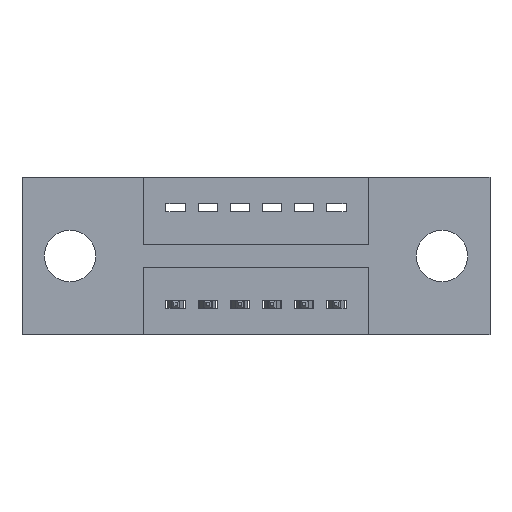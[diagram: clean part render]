
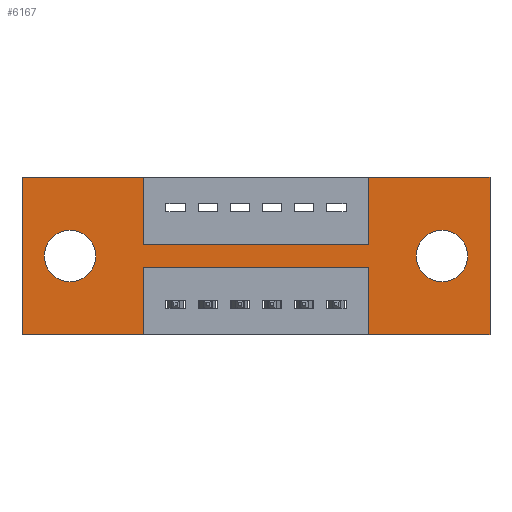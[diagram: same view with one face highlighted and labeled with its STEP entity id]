
A CAD part, front view. The second image highlights one B-rep face of the part: STEP entity #6167.
In plain terms, the highlighted planar face has unit normal (0, -1, 0).
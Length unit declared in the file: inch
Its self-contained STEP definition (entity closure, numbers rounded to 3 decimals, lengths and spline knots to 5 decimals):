
#45 = AXIS2_PLACEMENT_3D ( 'NONE', #7279, #2734, #5345 ) ;
#83 = CARTESIAN_POINT ( 'NONE',  ( 1.455, 0., 0. ) ) ;
#121 = ORIENTED_EDGE ( 'NONE', *, *, #7552, .F. ) ;
#159 = VECTOR ( 'NONE', #7605, 39.37008 ) ;
#226 = CARTESIAN_POINT ( 'NONE',  ( 1.0775, 0., -0.28 ) ) ;
#265 = FACE_BOUND ( 'NONE', #7285, .T. ) ;
#382 = CIRCLE ( 'NONE', #4432, 0.08 ) ;
#390 = ORIENTED_EDGE ( 'NONE', *, *, #767, .F. ) ;
#437 = ORIENTED_EDGE ( 'NONE', *, *, #5934, .F. ) ;
#606 = DIRECTION ( 'NONE',  ( 0., 0., 1. ) ) ;
#667 = DIRECTION ( 'NONE',  ( 0., 1., 0. ) ) ;
#767 = EDGE_CURVE ( 'NONE', #7581, #5680, #3666, .T. ) ;
#814 = ORIENTED_EDGE ( 'NONE', *, *, #2601, .F. ) ;
#1034 = CARTESIAN_POINT ( 'NONE',  ( 0.3775, 0., -0.21 ) ) ;
#1051 = PLANE ( 'NONE',  #6440 ) ;
#1087 = VERTEX_POINT ( 'NONE', #6138 ) ;
#1097 = DIRECTION ( 'NONE',  ( 0., 0., -1. ) ) ;
#1158 = DIRECTION ( 'NONE',  ( -1., 0., 0. ) ) ;
#1218 = ORIENTED_EDGE ( 'NONE', *, *, #6823, .F. ) ;
#1229 = VECTOR ( 'NONE', #1097, 39.37008 ) ;
#1241 = VECTOR ( 'NONE', #2586, 39.37008 ) ;
#1243 = VECTOR ( 'NONE', #2256, 39.37008 ) ;
#1257 = VECTOR ( 'NONE', #1158, 39.37008 ) ;
#1341 = EDGE_CURVE ( 'NONE', #1511, #5667, #7652, .T. ) ;
#1365 = CARTESIAN_POINT ( 'NONE',  ( 0.3775, 0., -0.49 ) ) ;
#1400 = DIRECTION ( 'NONE',  ( 0., 0., -1. ) ) ;
#1401 = VERTEX_POINT ( 'NONE', #8086 ) ;
#1511 = VERTEX_POINT ( 'NONE', #7092 ) ;
#1522 = DIRECTION ( 'NONE',  ( 0., 0., 1. ) ) ;
#1617 = VERTEX_POINT ( 'NONE', #7292 ) ;
#1715 = ORIENTED_EDGE ( 'NONE', *, *, #3439, .F. ) ;
#1744 = CARTESIAN_POINT ( 'NONE',  ( 0.1495, 0., -0.325 ) ) ;
#1856 = LINE ( 'NONE', #2813, #1243 ) ;
#1900 = LINE ( 'NONE', #2518, #1241 ) ;
#1903 = DIRECTION ( 'NONE',  ( 0., 0., -1. ) ) ;
#2095 = ORIENTED_EDGE ( 'NONE', *, *, #2577, .F. ) ;
#2156 = ORIENTED_EDGE ( 'NONE', *, *, #5410, .T. ) ;
#2192 = CIRCLE ( 'NONE', #5036, 0.08 ) ;
#2193 = CARTESIAN_POINT ( 'NONE',  ( 0.3775, 0., -0.21 ) ) ;
#2198 = CARTESIAN_POINT ( 'NONE',  ( 0., 0., 0. ) ) ;
#2256 = DIRECTION ( 'NONE',  ( -1., 0., 0. ) ) ;
#2380 = ORIENTED_EDGE ( 'NONE', *, *, #4853, .T. ) ;
#2443 = CARTESIAN_POINT ( 'NONE',  ( 1.0775, 0., -0.21 ) ) ;
#2518 = CARTESIAN_POINT ( 'NONE',  ( 0.3775, 0., -0.28 ) ) ;
#2527 = CARTESIAN_POINT ( 'NONE',  ( 0., 0., -0.49 ) ) ;
#2567 = LINE ( 'NONE', #2527, #6413 ) ;
#2577 = EDGE_CURVE ( 'NONE', #7084, #5293, #3788, .T. ) ;
#2586 = DIRECTION ( 'NONE',  ( 0., 0., -1. ) ) ;
#2598 = ORIENTED_EDGE ( 'NONE', *, *, #1341, .F. ) ;
#2601 = EDGE_CURVE ( 'NONE', #2740, #7581, #5428, .T. ) ;
#2621 = EDGE_LOOP ( 'NONE', ( #390, #814, #7301, #2862, #2598, #437, #121, #5266, #2095, #1715, #1218, #3570 ) ) ;
#2734 = DIRECTION ( 'NONE',  ( 0., 1., 0. ) ) ;
#2740 = VERTEX_POINT ( 'NONE', #1034 ) ;
#2776 = FACE_BOUND ( 'NONE', #6058, .T. ) ;
#2813 = CARTESIAN_POINT ( 'NONE',  ( 0.3775, 0., -0.28 ) ) ;
#2862 = ORIENTED_EDGE ( 'NONE', *, *, #6723, .F. ) ;
#2925 = ORIENTED_EDGE ( 'NONE', *, *, #5354, .T. ) ;
#3052 = VERTEX_POINT ( 'NONE', #1365 ) ;
#3074 = DIRECTION ( 'NONE',  ( 1., 0., 0. ) ) ;
#3151 = CARTESIAN_POINT ( 'NONE',  ( 0.1495, 0., -0.245 ) ) ;
#3234 = VERTEX_POINT ( 'NONE', #4937 ) ;
#3439 = EDGE_CURVE ( 'NONE', #6186, #7084, #2567, .T. ) ;
#3562 = VERTEX_POINT ( 'NONE', #4065 ) ;
#3570 = ORIENTED_EDGE ( 'NONE', *, *, #5876, .F. ) ;
#3621 = CIRCLE ( 'NONE', #45, 0.08 ) ;
#3666 = LINE ( 'NONE', #2443, #6799 ) ;
#3691 = VECTOR ( 'NONE', #3074, 39.37008 ) ;
#3788 = LINE ( 'NONE', #226, #7334 ) ;
#3817 = CARTESIAN_POINT ( 'NONE',  ( 0.1495, 0., -0.245 ) ) ;
#4065 = CARTESIAN_POINT ( 'NONE',  ( 1.3055, 0., -0.165 ) ) ;
#4267 = CARTESIAN_POINT ( 'NONE',  ( 0., 0., -0.49 ) ) ;
#4326 = AXIS2_PLACEMENT_3D ( 'NONE', #3817, #667, #5806 ) ;
#4333 = EDGE_CURVE ( 'NONE', #3562, #5982, #3621, .T. ) ;
#4432 = AXIS2_PLACEMENT_3D ( 'NONE', #3151, #7658, #606 ) ;
#4745 = CARTESIAN_POINT ( 'NONE',  ( 0., 0., 0. ) ) ;
#4789 = VERTEX_POINT ( 'NONE', #1744 ) ;
#4853 = EDGE_CURVE ( 'NONE', #5982, #3562, #2192, .T. ) ;
#4937 = CARTESIAN_POINT ( 'NONE',  ( 0.3775, 0., -0.28 ) ) ;
#5036 = AXIS2_PLACEMENT_3D ( 'NONE', #7853, #5084, #1400 ) ;
#5084 = DIRECTION ( 'NONE',  ( 0., 1., 0. ) ) ;
#5088 = VECTOR ( 'NONE', #1903, 39.37008 ) ;
#5141 = CARTESIAN_POINT ( 'NONE',  ( 1.3055, 0., -0.325 ) ) ;
#5266 = ORIENTED_EDGE ( 'NONE', *, *, #6476, .F. ) ;
#5293 = VERTEX_POINT ( 'NONE', #5736 ) ;
#5296 = LINE ( 'NONE', #83, #5088 ) ;
#5310 = LINE ( 'NONE', #6960, #159 ) ;
#5345 = DIRECTION ( 'NONE',  ( 0., 0., -1. ) ) ;
#5354 = EDGE_CURVE ( 'NONE', #1401, #4789, #8151, .T. ) ;
#5410 = EDGE_CURVE ( 'NONE', #4789, #1401, #382, .T. ) ;
#5428 = LINE ( 'NONE', #2193, #6622 ) ;
#5644 = CARTESIAN_POINT ( 'NONE',  ( 0., 0., 0. ) ) ;
#5667 = VERTEX_POINT ( 'NONE', #2198 ) ;
#5680 = VERTEX_POINT ( 'NONE', #6721 ) ;
#5736 = CARTESIAN_POINT ( 'NONE',  ( 1.0775, 0., -0.28 ) ) ;
#5806 = DIRECTION ( 'NONE',  ( 0., 0., 1. ) ) ;
#5814 = LINE ( 'NONE', #5644, #3691 ) ;
#5876 = EDGE_CURVE ( 'NONE', #5680, #1617, #5814, .T. ) ;
#5878 = DIRECTION ( 'NONE',  ( -1., 0., 0. ) ) ;
#5902 = DIRECTION ( 'NONE',  ( 0., 0., 1. ) ) ;
#5934 = EDGE_CURVE ( 'NONE', #3052, #1511, #7730, .T. ) ;
#5982 = VERTEX_POINT ( 'NONE', #5141 ) ;
#6058 = EDGE_LOOP ( 'NONE', ( #2925, #2156 ) ) ;
#6138 = CARTESIAN_POINT ( 'NONE',  ( 0.3775, 0., 0. ) ) ;
#6167 = ADVANCED_FACE ( 'NONE', ( #265, #2776, #6720 ), #1051, .T. ) ;
#6186 = VERTEX_POINT ( 'NONE', #7437 ) ;
#6191 = DIRECTION ( 'NONE',  ( 0., 0., -1. ) ) ;
#6313 = ORIENTED_EDGE ( 'NONE', *, *, #4333, .T. ) ;
#6413 = VECTOR ( 'NONE', #5878, 39.37008 ) ;
#6440 = AXIS2_PLACEMENT_3D ( 'NONE', #4267, #6864, #6191 ) ;
#6476 = EDGE_CURVE ( 'NONE', #5293, #3234, #1856, .T. ) ;
#6622 = VECTOR ( 'NONE', #7419, 39.37008 ) ;
#6657 = DIRECTION ( 'NONE',  ( 0., 0., 1. ) ) ;
#6720 = FACE_OUTER_BOUND ( 'NONE', #2621, .T. ) ;
#6721 = CARTESIAN_POINT ( 'NONE',  ( 1.0775, 0., 0. ) ) ;
#6723 = EDGE_CURVE ( 'NONE', #5667, #1087, #5310, .T. ) ;
#6792 = CARTESIAN_POINT ( 'NONE',  ( 1.0775, 0., -0.49 ) ) ;
#6799 = VECTOR ( 'NONE', #5902, 39.37008 ) ;
#6823 = EDGE_CURVE ( 'NONE', #1617, #6186, #5296, .T. ) ;
#6864 = DIRECTION ( 'NONE',  ( 0., -1., 0. ) ) ;
#6877 = CARTESIAN_POINT ( 'NONE',  ( 0.3775, 0., -0.21 ) ) ;
#6960 = CARTESIAN_POINT ( 'NONE',  ( 0., 0., 0. ) ) ;
#6995 = CARTESIAN_POINT ( 'NONE',  ( 0., 0., -0.49 ) ) ;
#7084 = VERTEX_POINT ( 'NONE', #6792 ) ;
#7092 = CARTESIAN_POINT ( 'NONE',  ( 0., 0., -0.49 ) ) ;
#7279 = CARTESIAN_POINT ( 'NONE',  ( 1.3055, 0., -0.245 ) ) ;
#7285 = EDGE_LOOP ( 'NONE', ( #6313, #2380 ) ) ;
#7292 = CARTESIAN_POINT ( 'NONE',  ( 1.455, 0., 0. ) ) ;
#7301 = ORIENTED_EDGE ( 'NONE', *, *, #8329, .F. ) ;
#7334 = VECTOR ( 'NONE', #6657, 39.37008 ) ;
#7419 = DIRECTION ( 'NONE',  ( 1., 0., 0. ) ) ;
#7437 = CARTESIAN_POINT ( 'NONE',  ( 1.455, 0., -0.49 ) ) ;
#7552 = EDGE_CURVE ( 'NONE', #3234, #3052, #1900, .T. ) ;
#7581 = VERTEX_POINT ( 'NONE', #7697 ) ;
#7605 = DIRECTION ( 'NONE',  ( 1., 0., 0. ) ) ;
#7652 = LINE ( 'NONE', #4745, #8346 ) ;
#7658 = DIRECTION ( 'NONE',  ( 0., 1., 0. ) ) ;
#7697 = CARTESIAN_POINT ( 'NONE',  ( 1.0775, 0., -0.21 ) ) ;
#7730 = LINE ( 'NONE', #6995, #1257 ) ;
#7800 = LINE ( 'NONE', #6877, #1229 ) ;
#7853 = CARTESIAN_POINT ( 'NONE',  ( 1.3055, 0., -0.245 ) ) ;
#8086 = CARTESIAN_POINT ( 'NONE',  ( 0.1495, 0., -0.165 ) ) ;
#8151 = CIRCLE ( 'NONE', #4326, 0.08 ) ;
#8329 = EDGE_CURVE ( 'NONE', #1087, #2740, #7800, .T. ) ;
#8346 = VECTOR ( 'NONE', #1522, 39.37008 ) ;
